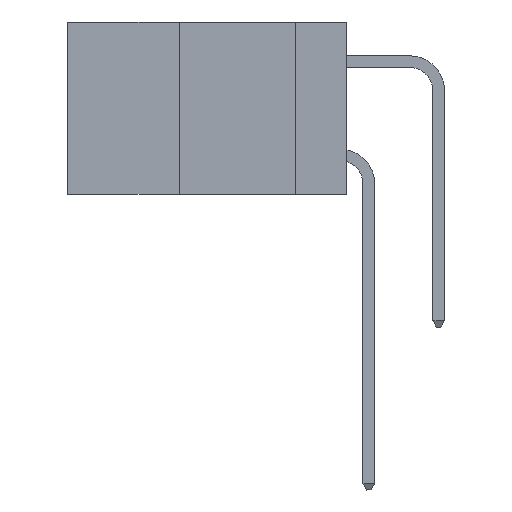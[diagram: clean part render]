
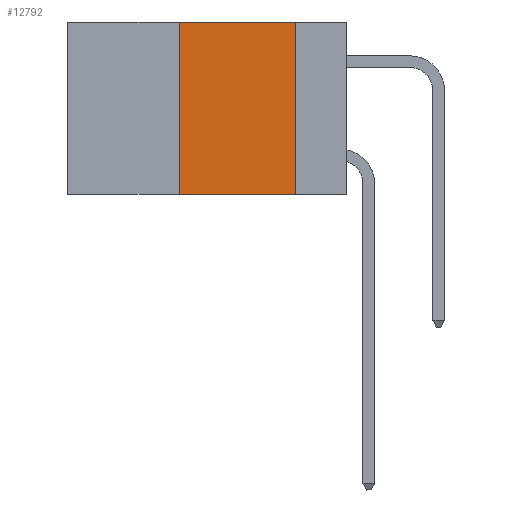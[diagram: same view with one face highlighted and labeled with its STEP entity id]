
A CAD part, left-side view. The second image highlights one B-rep face of the part: STEP entity #12792.
In plain terms, the highlighted planar face has unit normal (-1, 0, 0).
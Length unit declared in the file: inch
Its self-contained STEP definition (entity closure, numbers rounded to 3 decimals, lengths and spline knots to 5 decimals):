
#316 = AXIS2_PLACEMENT_3D ( 'NONE', #20434, #35735, #5279 ) ;
#1575 = ORIENTED_EDGE ( 'NONE', *, *, #29409, .F. ) ;
#5279 = DIRECTION ( 'NONE',  ( 0., 0., -1. ) ) ;
#7066 = CARTESIAN_POINT ( 'NONE',  ( 0., 0.11, 0. ) ) ;
#7658 = VERTEX_POINT ( 'NONE', #36380 ) ;
#9665 = EDGE_LOOP ( 'NONE', ( #24742, #16325, #1575, #16603 ) ) ;
#11321 = CARTESIAN_POINT ( 'NONE',  ( 0., 0.11, -0.37 ) ) ;
#11325 = VERTEX_POINT ( 'NONE', #37031 ) ;
#12792 = ADVANCED_FACE ( 'NONE', ( #28730 ), #38535, .F. ) ;
#13005 = DIRECTION ( 'NONE',  ( 0., 0., -1. ) ) ;
#13057 = VECTOR ( 'NONE', #13463, 39.37008 ) ;
#13463 = DIRECTION ( 'NONE',  ( 0., 0., 1. ) ) ;
#13806 = CARTESIAN_POINT ( 'NONE',  ( 0., 0.6, 0. ) ) ;
#16325 = ORIENTED_EDGE ( 'NONE', *, *, #33638, .F. ) ;
#16603 = ORIENTED_EDGE ( 'NONE', *, *, #23358, .T. ) ;
#18992 = DIRECTION ( 'NONE',  ( 0., -1., 0. ) ) ;
#19932 = VERTEX_POINT ( 'NONE', #11321 ) ;
#20434 = CARTESIAN_POINT ( 'NONE',  ( 0., 0.6, 0. ) ) ;
#22289 = CARTESIAN_POINT ( 'NONE',  ( 0., 0.36, 0. ) ) ;
#22364 = EDGE_CURVE ( 'NONE', #7658, #19932, #23162, .T. ) ;
#23162 = LINE ( 'NONE', #7066, #35917 ) ;
#23358 = EDGE_CURVE ( 'NONE', #11325, #19932, #32993, .T. ) ;
#24546 = LINE ( 'NONE', #30678, #13057 ) ;
#24742 = ORIENTED_EDGE ( 'NONE', *, *, #22364, .F. ) ;
#24954 = VECTOR ( 'NONE', #18992, 39.37008 ) ;
#28730 = FACE_OUTER_BOUND ( 'NONE', #9665, .T. ) ;
#29409 = EDGE_CURVE ( 'NONE', #11325, #31267, #24546, .T. ) ;
#29666 = VECTOR ( 'NONE', #38048, 39.37008 ) ;
#30678 = CARTESIAN_POINT ( 'NONE',  ( 0., 0.36, 0. ) ) ;
#30872 = CARTESIAN_POINT ( 'NONE',  ( 0., 0.6, -0.37 ) ) ;
#31267 = VERTEX_POINT ( 'NONE', #22289 ) ;
#32937 = LINE ( 'NONE', #13806, #29666 ) ;
#32993 = LINE ( 'NONE', #30872, #24954 ) ;
#33638 = EDGE_CURVE ( 'NONE', #31267, #7658, #32937, .T. ) ;
#35735 = DIRECTION ( 'NONE',  ( 1., 0., 0. ) ) ;
#35917 = VECTOR ( 'NONE', #13005, 39.37008 ) ;
#36380 = CARTESIAN_POINT ( 'NONE',  ( 0., 0.11, 0. ) ) ;
#37031 = CARTESIAN_POINT ( 'NONE',  ( 0., 0.36, -0.37 ) ) ;
#38048 = DIRECTION ( 'NONE',  ( 0., -1., 0. ) ) ;
#38535 = PLANE ( 'NONE',  #316 ) ;
